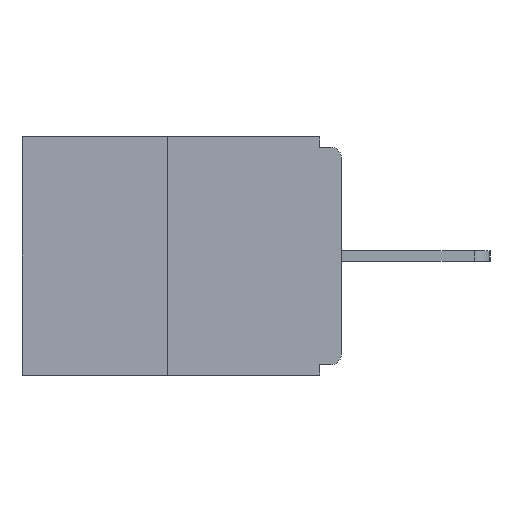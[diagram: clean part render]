
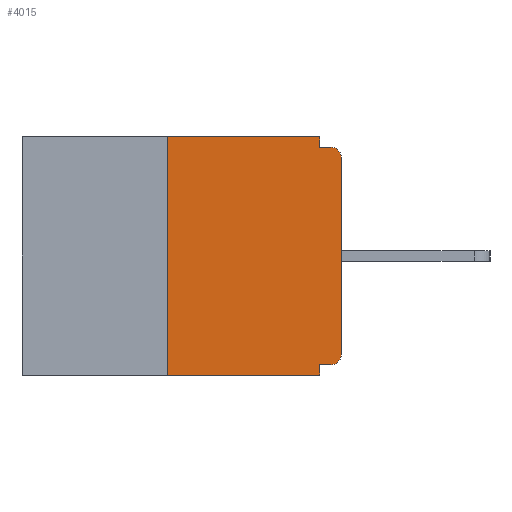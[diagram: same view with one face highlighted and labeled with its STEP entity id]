
A CAD part, left-side view. The second image highlights one B-rep face of the part: STEP entity #4015.
In plain terms, the highlighted planar face has unit normal (-1, 0, 0).
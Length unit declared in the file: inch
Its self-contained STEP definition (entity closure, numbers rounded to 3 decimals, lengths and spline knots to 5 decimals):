
#9 = EDGE_CURVE ( 'NONE', #14560, #17171, #15926, .T. ) ;
#207 = DIRECTION ( 'NONE',  ( 0., 0., -1. ) ) ;
#523 = EDGE_CURVE ( 'NONE', #14560, #6666, #7816, .T. ) ;
#524 = AXIS2_PLACEMENT_3D ( 'NONE', #17484, #7407, #3327 ) ;
#681 = DIRECTION ( 'NONE',  ( 0., 0., -1. ) ) ;
#693 = ORIENTED_EDGE ( 'NONE', *, *, #9, .T. ) ;
#704 = DIRECTION ( 'NONE',  ( 0., 0., 1. ) ) ;
#938 = CARTESIAN_POINT ( 'NONE',  ( 0., 0., -0.313 ) ) ;
#1004 = DIRECTION ( 'NONE',  ( 0., 0., 1. ) ) ;
#1279 = CARTESIAN_POINT ( 'NONE',  ( 0., 0.031, -0.328 ) ) ;
#1522 = ORIENTED_EDGE ( 'NONE', *, *, #12895, .T. ) ;
#1546 = CARTESIAN_POINT ( 'NONE',  ( 0., 0.015, -0.015 ) ) ;
#2228 = CARTESIAN_POINT ( 'NONE',  ( 0., 0.25, 0. ) ) ;
#2710 = CARTESIAN_POINT ( 'NONE',  ( 0., 0., -0.328 ) ) ;
#2744 = EDGE_CURVE ( 'NONE', #10537, #14084, #10885, .T. ) ;
#2746 = CARTESIAN_POINT ( 'NONE',  ( 0., 0.015, -0.328 ) ) ;
#2776 = VECTOR ( 'NONE', #3244, 39.37008 ) ;
#3244 = DIRECTION ( 'NONE',  ( 0., 1., 0. ) ) ;
#3327 = DIRECTION ( 'NONE',  ( 0., 0., -1. ) ) ;
#3516 = ORIENTED_EDGE ( 'NONE', *, *, #13010, .T. ) ;
#3518 = CARTESIAN_POINT ( 'NONE',  ( 0., 0.031, 0. ) ) ;
#3574 = VECTOR ( 'NONE', #4431, 39.37008 ) ;
#4015 = ADVANCED_FACE ( 'NONE', ( #18649 ), #11487, .F. ) ;
#4431 = DIRECTION ( 'NONE',  ( 0., -1., 0. ) ) ;
#4586 = EDGE_CURVE ( 'NONE', #14495, #17171, #7491, .T. ) ;
#4856 = ORIENTED_EDGE ( 'NONE', *, *, #11148, .F. ) ;
#4958 = EDGE_CURVE ( 'NONE', #14084, #12821, #5859, .T. ) ;
#5577 = DIRECTION ( 'NONE',  ( 0., -1., 0. ) ) ;
#5647 = CARTESIAN_POINT ( 'NONE',  ( 0., 0.031, -0.015 ) ) ;
#5859 = LINE ( 'NONE', #11633, #13141 ) ;
#6197 = VERTEX_POINT ( 'NONE', #2746 ) ;
#6450 = CARTESIAN_POINT ( 'NONE',  ( 0., 0.015, -0.313 ) ) ;
#6469 = CARTESIAN_POINT ( 'NONE',  ( 0., 0.031, 0. ) ) ;
#6490 = VECTOR ( 'NONE', #207, 39.37008 ) ;
#6505 = CARTESIAN_POINT ( 'NONE',  ( 0., 0.031, -0.343 ) ) ;
#6666 = VERTEX_POINT ( 'NONE', #17343 ) ;
#6670 = ORIENTED_EDGE ( 'NONE', *, *, #4586, .F. ) ;
#7080 = CARTESIAN_POINT ( 'NONE',  ( 0., 0.46, -0.343 ) ) ;
#7309 = ORIENTED_EDGE ( 'NONE', *, *, #18024, .T. ) ;
#7407 = DIRECTION ( 'NONE',  ( -1., 0., 0. ) ) ;
#7491 = LINE ( 'NONE', #13244, #6490 ) ;
#7590 = VERTEX_POINT ( 'NONE', #13283 ) ;
#7704 = LINE ( 'NONE', #13649, #15431 ) ;
#7778 = CIRCLE ( 'NONE', #16499, 0.015 ) ;
#7816 = LINE ( 'NONE', #2228, #14080 ) ;
#8547 = CARTESIAN_POINT ( 'NONE',  ( 0., 0.25, -0.343 ) ) ;
#8555 = CARTESIAN_POINT ( 'NONE',  ( 0., 0.46, 0. ) ) ;
#8674 = CIRCLE ( 'NONE', #524, 0.015 ) ;
#9636 = ORIENTED_EDGE ( 'NONE', *, *, #16095, .F. ) ;
#9898 = LINE ( 'NONE', #10078, #15241 ) ;
#10078 = CARTESIAN_POINT ( 'NONE',  ( 0., 0.46, 0. ) ) ;
#10537 = VERTEX_POINT ( 'NONE', #6469 ) ;
#10885 = LINE ( 'NONE', #3518, #17913 ) ;
#11148 = EDGE_CURVE ( 'NONE', #6666, #10537, #9898, .T. ) ;
#11487 = PLANE ( 'NONE',  #13468 ) ;
#11633 = CARTESIAN_POINT ( 'NONE',  ( 0., 0., -0.015 ) ) ;
#12219 = DIRECTION ( 'NONE',  ( -1., 0., 0. ) ) ;
#12821 = VERTEX_POINT ( 'NONE', #1546 ) ;
#12895 = EDGE_CURVE ( 'NONE', #7590, #12821, #8674, .T. ) ;
#13010 = EDGE_CURVE ( 'NONE', #6197, #17333, #7778, .T. ) ;
#13141 = VECTOR ( 'NONE', #5577, 39.37008 ) ;
#13244 = CARTESIAN_POINT ( 'NONE',  ( 0., 0.031, -0.343 ) ) ;
#13283 = CARTESIAN_POINT ( 'NONE',  ( 0., 0., -0.03 ) ) ;
#13468 = AXIS2_PLACEMENT_3D ( 'NONE', #8555, #15979, #14477 ) ;
#13649 = CARTESIAN_POINT ( 'NONE',  ( 0., 0., 0. ) ) ;
#14080 = VECTOR ( 'NONE', #1004, 39.37008 ) ;
#14084 = VERTEX_POINT ( 'NONE', #5647 ) ;
#14130 = DIRECTION ( 'NONE',  ( 0., -1., 0. ) ) ;
#14477 = DIRECTION ( 'NONE',  ( 0., 0., -1. ) ) ;
#14495 = VERTEX_POINT ( 'NONE', #1279 ) ;
#14560 = VERTEX_POINT ( 'NONE', #8547 ) ;
#14903 = ORIENTED_EDGE ( 'NONE', *, *, #4958, .F. ) ;
#15241 = VECTOR ( 'NONE', #14130, 39.37008 ) ;
#15431 = VECTOR ( 'NONE', #704, 39.37008 ) ;
#15632 = LINE ( 'NONE', #2710, #2776 ) ;
#15926 = LINE ( 'NONE', #7080, #3574 ) ;
#15979 = DIRECTION ( 'NONE',  ( 1., 0., 0. ) ) ;
#16095 = EDGE_CURVE ( 'NONE', #6197, #14495, #15632, .T. ) ;
#16499 = AXIS2_PLACEMENT_3D ( 'NONE', #6450, #12219, #16722 ) ;
#16722 = DIRECTION ( 'NONE',  ( 0., 0., -1. ) ) ;
#17171 = VERTEX_POINT ( 'NONE', #6505 ) ;
#17333 = VERTEX_POINT ( 'NONE', #938 ) ;
#17343 = CARTESIAN_POINT ( 'NONE',  ( 0., 0.25, 0. ) ) ;
#17459 = ORIENTED_EDGE ( 'NONE', *, *, #523, .F. ) ;
#17484 = CARTESIAN_POINT ( 'NONE',  ( 0., 0.015, -0.03 ) ) ;
#17792 = ORIENTED_EDGE ( 'NONE', *, *, #2744, .F. ) ;
#17913 = VECTOR ( 'NONE', #681, 39.37008 ) ;
#18024 = EDGE_CURVE ( 'NONE', #17333, #7590, #7704, .T. ) ;
#18498 = EDGE_LOOP ( 'NONE', ( #4856, #17459, #693, #6670, #9636, #3516, #7309, #1522, #14903, #17792 ) ) ;
#18649 = FACE_OUTER_BOUND ( 'NONE', #18498, .T. ) ;
